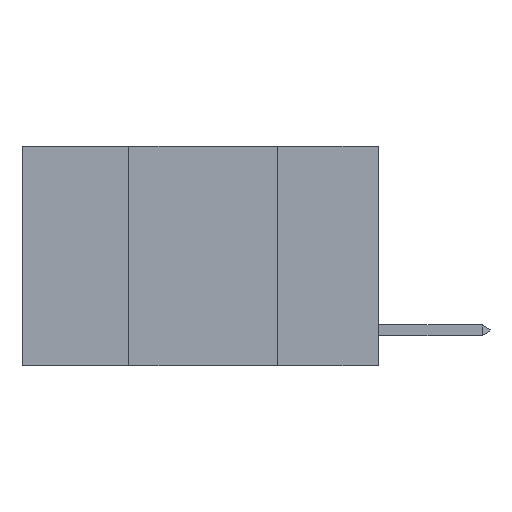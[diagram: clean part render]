
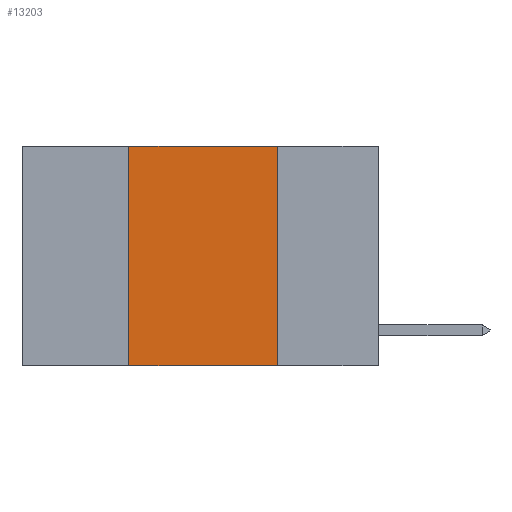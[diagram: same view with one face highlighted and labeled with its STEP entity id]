
A CAD part, left-side view. The second image highlights one B-rep face of the part: STEP entity #13203.
In plain terms, the highlighted planar face has unit normal (-1, 0, 0).
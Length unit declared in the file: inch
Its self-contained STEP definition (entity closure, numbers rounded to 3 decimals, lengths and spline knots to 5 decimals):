
#525 = DIRECTION ( 'NONE',  ( 0., 0., -1. ) ) ;
#1425 = EDGE_LOOP ( 'NONE', ( #6892, #10733, #11190, #14999 ) ) ;
#2876 = EDGE_CURVE ( 'NONE', #2925, #18561, #8546, .T. ) ;
#2925 = VERTEX_POINT ( 'NONE', #11163 ) ;
#3326 = CARTESIAN_POINT ( 'NONE',  ( 0., 0.42, 0. ) ) ;
#4172 = FACE_OUTER_BOUND ( 'NONE', #1425, .T. ) ;
#4313 = DIRECTION ( 'NONE',  ( 0., -1., 0. ) ) ;
#5430 = EDGE_CURVE ( 'NONE', #16459, #18561, #13835, .T. ) ;
#5737 = LINE ( 'NONE', #18765, #12948 ) ;
#5790 = CARTESIAN_POINT ( 'NONE',  ( 0., 0.6, -0.37 ) ) ;
#6177 = VECTOR ( 'NONE', #4313, 39.37008 ) ;
#6439 = CARTESIAN_POINT ( 'NONE',  ( 0., 0.17, -0.37 ) ) ;
#6892 = ORIENTED_EDGE ( 'NONE', *, *, #2876, .F. ) ;
#7899 = PLANE ( 'NONE',  #18289 ) ;
#8078 = VECTOR ( 'NONE', #11041, 39.37008 ) ;
#8089 = CARTESIAN_POINT ( 'NONE',  ( 0., 0.17, 0. ) ) ;
#8426 = EDGE_CURVE ( 'NONE', #16459, #16170, #5737, .T. ) ;
#8546 = LINE ( 'NONE', #8089, #8078 ) ;
#9342 = DIRECTION ( 'NONE',  ( 1., 0., 0. ) ) ;
#9777 = CARTESIAN_POINT ( 'NONE',  ( 0., 0.42, -0.37 ) ) ;
#10248 = DIRECTION ( 'NONE',  ( 0., 0., 1. ) ) ;
#10733 = ORIENTED_EDGE ( 'NONE', *, *, #17620, .F. ) ;
#11041 = DIRECTION ( 'NONE',  ( 0., 0., -1. ) ) ;
#11076 = VECTOR ( 'NONE', #18222, 39.37008 ) ;
#11163 = CARTESIAN_POINT ( 'NONE',  ( 0., 0.17, 0. ) ) ;
#11190 = ORIENTED_EDGE ( 'NONE', *, *, #8426, .F. ) ;
#11972 = LINE ( 'NONE', #15439, #11076 ) ;
#12948 = VECTOR ( 'NONE', #10248, 39.37008 ) ;
#13203 = ADVANCED_FACE ( 'NONE', ( #4172 ), #7899, .F. ) ;
#13835 = LINE ( 'NONE', #5790, #6177 ) ;
#14999 = ORIENTED_EDGE ( 'NONE', *, *, #5430, .T. ) ;
#15439 = CARTESIAN_POINT ( 'NONE',  ( 0., 0.6, 0. ) ) ;
#16170 = VERTEX_POINT ( 'NONE', #3326 ) ;
#16459 = VERTEX_POINT ( 'NONE', #9777 ) ;
#17620 = EDGE_CURVE ( 'NONE', #16170, #2925, #11972, .T. ) ;
#17899 = CARTESIAN_POINT ( 'NONE',  ( 0., 0.6, 0. ) ) ;
#18222 = DIRECTION ( 'NONE',  ( 0., -1., 0. ) ) ;
#18289 = AXIS2_PLACEMENT_3D ( 'NONE', #17899, #9342, #525 ) ;
#18561 = VERTEX_POINT ( 'NONE', #6439 ) ;
#18765 = CARTESIAN_POINT ( 'NONE',  ( 0., 0.42, 0. ) ) ;
